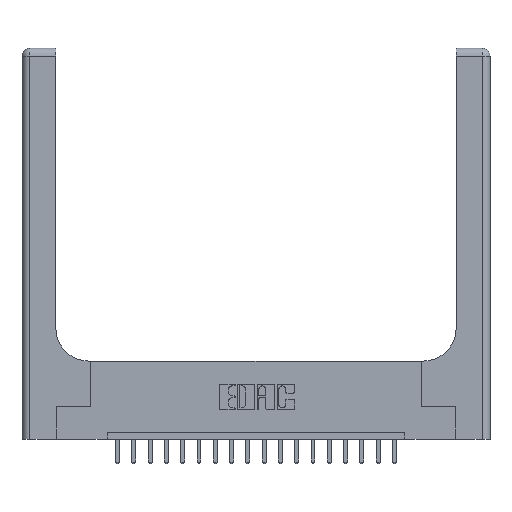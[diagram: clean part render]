
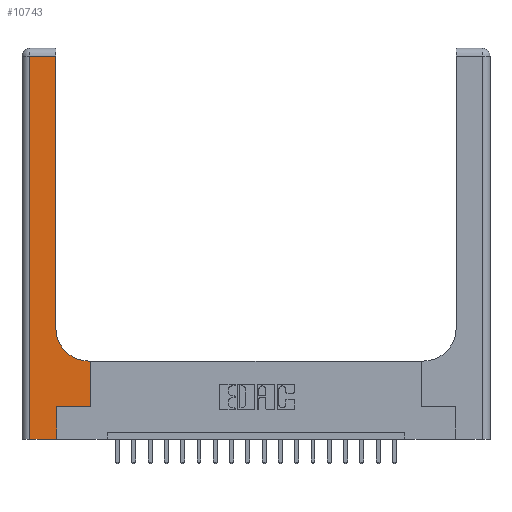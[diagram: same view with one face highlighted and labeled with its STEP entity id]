
A CAD part, top view. The second image highlights one B-rep face of the part: STEP entity #10743.
In plain terms, the highlighted planar face has unit normal (0, 0, 1).
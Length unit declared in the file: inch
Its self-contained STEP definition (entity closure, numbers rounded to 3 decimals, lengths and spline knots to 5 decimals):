
#382 = DIRECTION ( 'NONE',  ( -1., 0., 0. ) ) ;
#684 = VERTEX_POINT ( 'NONE', #10683 ) ;
#689 = ORIENTED_EDGE ( 'NONE', *, *, #12334, .T. ) ;
#1646 = LINE ( 'NONE', #18020, #14467 ) ;
#1741 = ORIENTED_EDGE ( 'NONE', *, *, #16531, .T. ) ;
#2181 = CARTESIAN_POINT ( 'NONE',  ( 0., 0., 0.37 ) ) ;
#2260 = DIRECTION ( 'NONE',  ( 1., 0., 0. ) ) ;
#2728 = VECTOR ( 'NONE', #12992, 39.37008 ) ;
#3132 = LINE ( 'NONE', #5470, #12405 ) ;
#3441 = CARTESIAN_POINT ( 'NONE',  ( 0.26, 2.94, 0.37 ) ) ;
#3826 = CARTESIAN_POINT ( 'NONE',  ( 0.51, 0.6, 0.37 ) ) ;
#4088 = DIRECTION ( 'NONE',  ( -1., 0., 0. ) ) ;
#4255 = EDGE_CURVE ( 'NONE', #684, #19418, #14809, .T. ) ;
#4619 = LINE ( 'NONE', #2181, #2728 ) ;
#4922 = CARTESIAN_POINT ( 'NONE',  ( 0.26, 3., 0.37 ) ) ;
#4954 = ORIENTED_EDGE ( 'NONE', *, *, #5563, .T. ) ;
#5027 = CARTESIAN_POINT ( 'NONE',  ( 0.528, 0.25, 0.37 ) ) ;
#5159 = DIRECTION ( 'NONE',  ( 0., 1., 0. ) ) ;
#5259 = EDGE_CURVE ( 'NONE', #16378, #14261, #3132, .T. ) ;
#5470 = CARTESIAN_POINT ( 'NONE',  ( 0.26, 0.6, 0.37 ) ) ;
#5530 = EDGE_CURVE ( 'NONE', #19418, #15828, #10732, .T. ) ;
#5563 = EDGE_CURVE ( 'NONE', #18948, #18918, #17132, .T. ) ;
#5663 = AXIS2_PLACEMENT_3D ( 'NONE', #8287, #18980, #15699 ) ;
#5998 = VECTOR ( 'NONE', #18976, 39.37008 ) ;
#6292 = CIRCLE ( 'NONE', #16306, 0.25 ) ;
#6812 = CARTESIAN_POINT ( 'NONE',  ( 0.265, 0., 0.37 ) ) ;
#7787 = CARTESIAN_POINT ( 'NONE',  ( 0.265, 0.25, 0.37 ) ) ;
#8211 = VERTEX_POINT ( 'NONE', #9024 ) ;
#8287 = CARTESIAN_POINT ( 'NONE',  ( 0., 3., 0.37 ) ) ;
#8543 = CARTESIAN_POINT ( 'NONE',  ( 0.528, 0.6, 0.37 ) ) ;
#9024 = CARTESIAN_POINT ( 'NONE',  ( 0.265, 0., 0.37 ) ) ;
#9511 = VECTOR ( 'NONE', #382, 39.37008 ) ;
#9837 = EDGE_LOOP ( 'NONE', ( #18946, #15847, #1741, #689, #12473, #4954, #17264, #14614, #12375 ) ) ;
#10683 = CARTESIAN_POINT ( 'NONE',  ( 0.26, 0.85, 0.37 ) ) ;
#10732 = LINE ( 'NONE', #17182, #9511 ) ;
#10743 = ADVANCED_FACE ( 'NONE', ( #14417 ), #12640, .F. ) ;
#10949 = VECTOR ( 'NONE', #5159, 39.37008 ) ;
#11083 = VERTEX_POINT ( 'NONE', #18484 ) ;
#11238 = VECTOR ( 'NONE', #15834, 39.37008 ) ;
#11324 = EDGE_CURVE ( 'NONE', #14261, #684, #6292, .T. ) ;
#11353 = CARTESIAN_POINT ( 'NONE',  ( 0.51, 0.85, 0.37 ) ) ;
#11450 = CARTESIAN_POINT ( 'NONE',  ( 0.265, 0.25, 0.37 ) ) ;
#11998 = DIRECTION ( 'NONE',  ( 0., -1., 0. ) ) ;
#12334 = EDGE_CURVE ( 'NONE', #11083, #8211, #4619, .T. ) ;
#12375 = ORIENTED_EDGE ( 'NONE', *, *, #11324, .T. ) ;
#12376 = CARTESIAN_POINT ( 'NONE',  ( 0.06, 2.94, 0.37 ) ) ;
#12405 = VECTOR ( 'NONE', #4088, 39.37008 ) ;
#12473 = ORIENTED_EDGE ( 'NONE', *, *, #13018, .T. ) ;
#12640 = PLANE ( 'NONE',  #5663 ) ;
#12853 = LINE ( 'NONE', #5027, #10949 ) ;
#12992 = DIRECTION ( 'NONE',  ( 1., 0., 0. ) ) ;
#13018 = EDGE_CURVE ( 'NONE', #8211, #18948, #15069, .T. ) ;
#14186 = DIRECTION ( 'NONE',  ( 1., 0., 0. ) ) ;
#14261 = VERTEX_POINT ( 'NONE', #3826 ) ;
#14417 = FACE_OUTER_BOUND ( 'NONE', #9837, .T. ) ;
#14467 = VECTOR ( 'NONE', #11998, 39.37008 ) ;
#14614 = ORIENTED_EDGE ( 'NONE', *, *, #5259, .T. ) ;
#14699 = EDGE_CURVE ( 'NONE', #18918, #16378, #12853, .T. ) ;
#14809 = LINE ( 'NONE', #4922, #11238 ) ;
#15069 = LINE ( 'NONE', #6812, #5998 ) ;
#15256 = VECTOR ( 'NONE', #14186, 39.37008 ) ;
#15627 = CARTESIAN_POINT ( 'NONE',  ( 0.528, 0.25, 0.37 ) ) ;
#15699 = DIRECTION ( 'NONE',  ( -1., 0., 0. ) ) ;
#15828 = VERTEX_POINT ( 'NONE', #12376 ) ;
#15834 = DIRECTION ( 'NONE',  ( 0., 1., 0. ) ) ;
#15847 = ORIENTED_EDGE ( 'NONE', *, *, #5530, .T. ) ;
#16306 = AXIS2_PLACEMENT_3D ( 'NONE', #11353, #18956, #2260 ) ;
#16378 = VERTEX_POINT ( 'NONE', #8543 ) ;
#16531 = EDGE_CURVE ( 'NONE', #15828, #11083, #1646, .T. ) ;
#17132 = LINE ( 'NONE', #7787, #15256 ) ;
#17182 = CARTESIAN_POINT ( 'NONE',  ( 0., 2.94, 0.37 ) ) ;
#17264 = ORIENTED_EDGE ( 'NONE', *, *, #14699, .T. ) ;
#18020 = CARTESIAN_POINT ( 'NONE',  ( 0.06, 3., 0.37 ) ) ;
#18484 = CARTESIAN_POINT ( 'NONE',  ( 0.06, 0., 0.37 ) ) ;
#18918 = VERTEX_POINT ( 'NONE', #15627 ) ;
#18946 = ORIENTED_EDGE ( 'NONE', *, *, #4255, .T. ) ;
#18948 = VERTEX_POINT ( 'NONE', #11450 ) ;
#18956 = DIRECTION ( 'NONE',  ( 0., 0., -1. ) ) ;
#18976 = DIRECTION ( 'NONE',  ( 0., 1., 0. ) ) ;
#18980 = DIRECTION ( 'NONE',  ( 0., 0., -1. ) ) ;
#19418 = VERTEX_POINT ( 'NONE', #3441 ) ;
